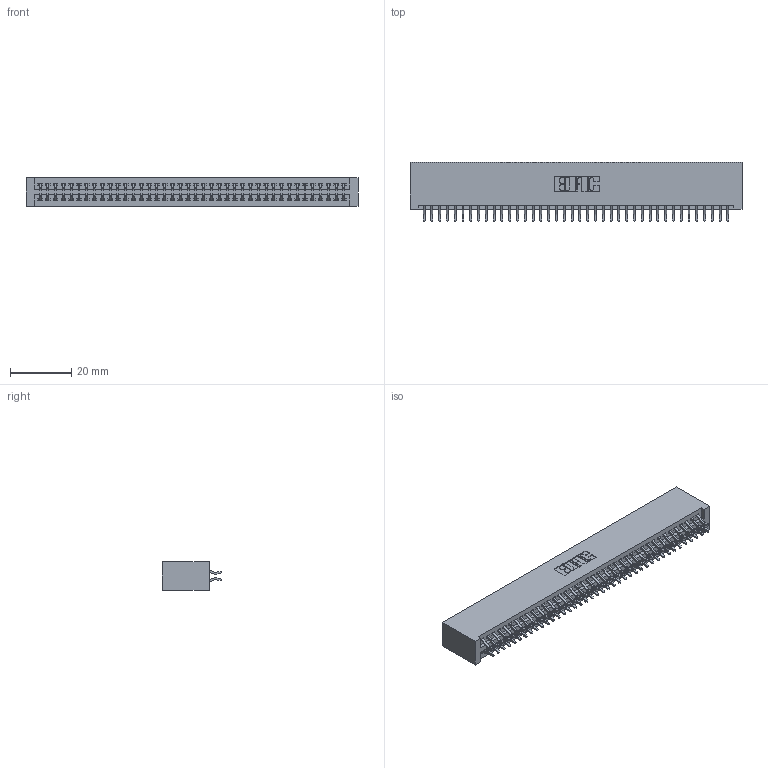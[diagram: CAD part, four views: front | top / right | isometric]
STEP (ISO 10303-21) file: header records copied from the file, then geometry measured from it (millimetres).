
FILE_DESCRIPTION (( 'STEP AP203' ), '1' );
FILE_NAME ('345-080-556-201.STEP', '2018-10-03T18:52:22', ( '' ), ( '' ), 'SwSTEP 2.0', 'SolidWorks 2016', '' );
FILE_SCHEMA (( 'CONFIG_CONTROL_DESIGN' ));
Length unit declared in the file: inch
Products named in the file (3): 345 Part_No Mounting Lugs; 345-080-556-201; 345-292-001_556 Tail
Assembly tree (81 placements, depth 2):
  345-080-556-201
    345 Part_No Mounting Lugs
    345-292-001_556 Tail  x80
Bounding box: 108.2 x 19.24 x 9.4 mm (x, y, z)
Volume: 11105.2 mm3; surface area: 16609.9 mm2
Topology: 81 solids, 81 shells, 4598 faces, 13677 edges, 9010 vertices
Faces by surface type: plane 3036, cylinder 1562
Entity records: 31597 total; most frequent: CARTESIAN_POINT 5312, ORIENTED_EDGE 5234, DIRECTION 4669, EDGE_CURVE 2617, LINE 2325, VECTOR 2325, VERTEX_POINT 1742, AXIS2_PLACEMENT_3D 1172
